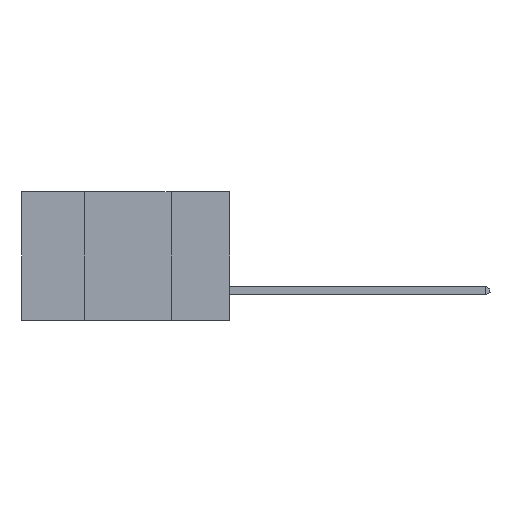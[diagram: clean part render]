
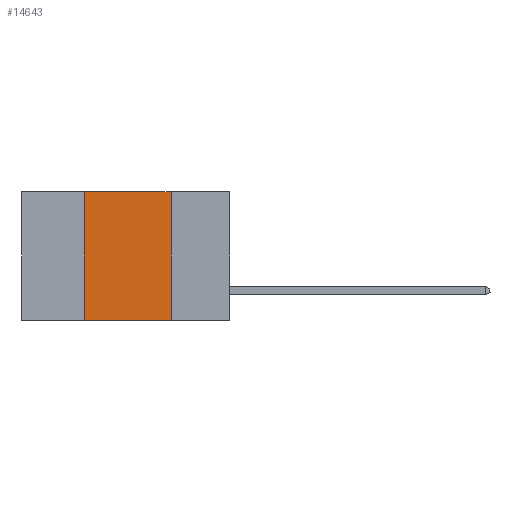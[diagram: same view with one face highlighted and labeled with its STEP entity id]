
A CAD part, left-side view. The second image highlights one B-rep face of the part: STEP entity #14643.
In plain terms, the highlighted planar face has unit normal (-1, 0, 0).
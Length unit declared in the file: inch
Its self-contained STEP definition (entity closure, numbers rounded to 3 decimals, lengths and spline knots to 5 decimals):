
#424 = VERTEX_POINT ( 'NONE', #11507 ) ;
#999 = VECTOR ( 'NONE', #3599, 39.37008 ) ;
#1520 = EDGE_LOOP ( 'NONE', ( #13183, #6483, #16997, #4485 ) ) ;
#2296 = CARTESIAN_POINT ( 'NONE',  ( 0., 0.6, -0.37 ) ) ;
#2479 = DIRECTION ( 'NONE',  ( 0., -1., 0. ) ) ;
#2502 = LINE ( 'NONE', #15240, #12192 ) ;
#3126 = DIRECTION ( 'NONE',  ( 0., 0., -1. ) ) ;
#3599 = DIRECTION ( 'NONE',  ( 0., 0., 1. ) ) ;
#3675 = VERTEX_POINT ( 'NONE', #11236 ) ;
#4215 = CARTESIAN_POINT ( 'NONE',  ( 0., 0.42, -0.37 ) ) ;
#4485 = ORIENTED_EDGE ( 'NONE', *, *, #15102, .T. ) ;
#6483 = ORIENTED_EDGE ( 'NONE', *, *, #16964, .F. ) ;
#7125 = PLANE ( 'NONE',  #10468 ) ;
#7316 = CARTESIAN_POINT ( 'NONE',  ( 0., 0.6, 0. ) ) ;
#8428 = DIRECTION ( 'NONE',  ( 0., -1., 0. ) ) ;
#9117 = CARTESIAN_POINT ( 'NONE',  ( 0., 0.42, 0. ) ) ;
#9775 = LINE ( 'NONE', #2296, #14270 ) ;
#10468 = AXIS2_PLACEMENT_3D ( 'NONE', #7316, #11222, #3126 ) ;
#11222 = DIRECTION ( 'NONE',  ( 1., 0., 0. ) ) ;
#11236 = CARTESIAN_POINT ( 'NONE',  ( 0., 0.17, 0. ) ) ;
#11507 = CARTESIAN_POINT ( 'NONE',  ( 0., 0.42, 0. ) ) ;
#11650 = VERTEX_POINT ( 'NONE', #11852 ) ;
#11665 = EDGE_CURVE ( 'NONE', #14093, #424, #15673, .T. ) ;
#11852 = CARTESIAN_POINT ( 'NONE',  ( 0., 0.17, -0.37 ) ) ;
#12119 = EDGE_CURVE ( 'NONE', #3675, #11650, #13934, .T. ) ;
#12192 = VECTOR ( 'NONE', #8428, 39.37008 ) ;
#12584 = FACE_OUTER_BOUND ( 'NONE', #1520, .T. ) ;
#13183 = ORIENTED_EDGE ( 'NONE', *, *, #12119, .F. ) ;
#13306 = VECTOR ( 'NONE', #17270, 39.37008 ) ;
#13934 = LINE ( 'NONE', #15797, #13306 ) ;
#14093 = VERTEX_POINT ( 'NONE', #4215 ) ;
#14270 = VECTOR ( 'NONE', #2479, 39.37008 ) ;
#14643 = ADVANCED_FACE ( 'NONE', ( #12584 ), #7125, .F. ) ;
#15102 = EDGE_CURVE ( 'NONE', #14093, #11650, #9775, .T. ) ;
#15240 = CARTESIAN_POINT ( 'NONE',  ( 0., 0.6, 0. ) ) ;
#15673 = LINE ( 'NONE', #9117, #999 ) ;
#15797 = CARTESIAN_POINT ( 'NONE',  ( 0., 0.17, 0. ) ) ;
#16964 = EDGE_CURVE ( 'NONE', #424, #3675, #2502, .T. ) ;
#16997 = ORIENTED_EDGE ( 'NONE', *, *, #11665, .F. ) ;
#17270 = DIRECTION ( 'NONE',  ( 0., 0., -1. ) ) ;
